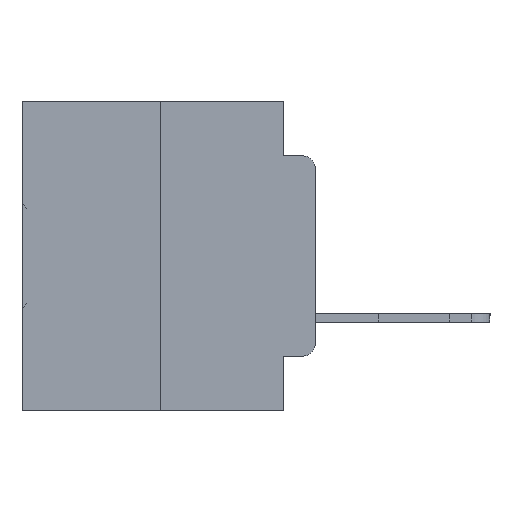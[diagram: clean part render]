
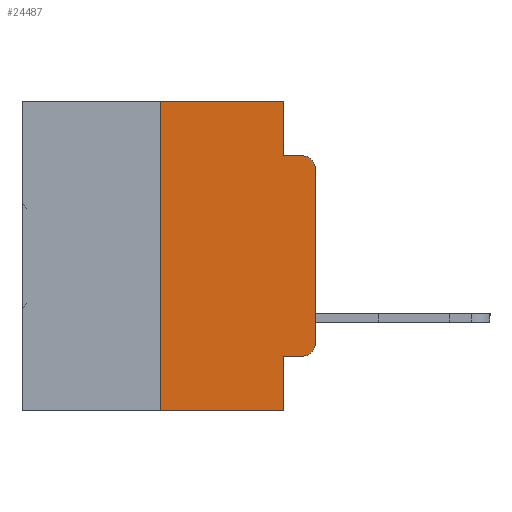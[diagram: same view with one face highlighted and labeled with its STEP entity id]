
A CAD part, left-side view. The second image highlights one B-rep face of the part: STEP entity #24487.
In plain terms, the highlighted planar face has unit normal (-1, 0, 0).
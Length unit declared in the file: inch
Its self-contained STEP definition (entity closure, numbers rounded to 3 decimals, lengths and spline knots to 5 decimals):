
#37 = VERTEX_POINT ( 'NONE', #17748 ) ;
#330 = DIRECTION ( 'NONE',  ( 0., 0., 1. ) ) ;
#816 = DIRECTION ( 'NONE',  ( 1., 0., 0. ) ) ;
#1724 = VECTOR ( 'NONE', #330, 39.37008 ) ;
#1955 = LINE ( 'NONE', #27634, #27703 ) ;
#2617 = CARTESIAN_POINT ( 'NONE',  ( 0., 0., -0.3915 ) ) ;
#2791 = LINE ( 'NONE', #24488, #22580 ) ;
#3688 = VERTEX_POINT ( 'NONE', #6544 ) ;
#3793 = FACE_OUTER_BOUND ( 'NONE', #29259, .T. ) ;
#4021 = ORIENTED_EDGE ( 'NONE', *, *, #22853, .F. ) ;
#4313 = VERTEX_POINT ( 'NONE', #27003 ) ;
#4497 = DIRECTION ( 'NONE',  ( 0., -1., 0. ) ) ;
#4817 = AXIS2_PLACEMENT_3D ( 'NONE', #11892, #29883, #14508 ) ;
#4866 = VERTEX_POINT ( 'NONE', #28330 ) ;
#6233 = CARTESIAN_POINT ( 'NONE',  ( 0., 0.473, -0.5 ) ) ;
#6544 = CARTESIAN_POINT ( 'NONE',  ( 0., 0.02, -0.4115 ) ) ;
#6559 = DIRECTION ( 'NONE',  ( 0., -1., 0. ) ) ;
#6731 = DIRECTION ( 'NONE',  ( -1., 0., 0. ) ) ;
#6744 = CARTESIAN_POINT ( 'NONE',  ( 0., 0.051, 0. ) ) ;
#7440 = LINE ( 'NONE', #6744, #33087 ) ;
#7523 = VECTOR ( 'NONE', #4497, 39.37008 ) ;
#8477 = EDGE_CURVE ( 'NONE', #4866, #23274, #1955, .T. ) ;
#9270 = DIRECTION ( 'NONE',  ( 0., 0., -1. ) ) ;
#9688 = VECTOR ( 'NONE', #19151, 39.37008 ) ;
#10139 = LINE ( 'NONE', #18176, #29871 ) ;
#10166 = EDGE_CURVE ( 'NONE', #4313, #20481, #10139, .T. ) ;
#10499 = ORIENTED_EDGE ( 'NONE', *, *, #17153, .F. ) ;
#10943 = LINE ( 'NONE', #18436, #1724 ) ;
#11037 = EDGE_CURVE ( 'NONE', #4313, #23274, #29813, .T. ) ;
#11892 = CARTESIAN_POINT ( 'NONE',  ( 0., 0.02, -0.1085 ) ) ;
#13663 = CARTESIAN_POINT ( 'NONE',  ( 0., 0.473, 0. ) ) ;
#13836 = CIRCLE ( 'NONE', #31294, 0.02 ) ;
#14319 = ORIENTED_EDGE ( 'NONE', *, *, #10166, .F. ) ;
#14508 = DIRECTION ( 'NONE',  ( 0., 0., -1. ) ) ;
#14827 = DIRECTION ( 'NONE',  ( 0., 0., -1. ) ) ;
#15124 = ORIENTED_EDGE ( 'NONE', *, *, #8477, .F. ) ;
#17153 = EDGE_CURVE ( 'NONE', #31834, #23799, #7440, .T. ) ;
#17427 = LINE ( 'NONE', #29294, #9688 ) ;
#17651 = ORIENTED_EDGE ( 'NONE', *, *, #28085, .T. ) ;
#17748 = CARTESIAN_POINT ( 'NONE',  ( 0., 0.02, -0.0885 ) ) ;
#17864 = ORIENTED_EDGE ( 'NONE', *, *, #11037, .T. ) ;
#18003 = ORIENTED_EDGE ( 'NONE', *, *, #25762, .T. ) ;
#18176 = CARTESIAN_POINT ( 'NONE',  ( 0., 0.25, 0. ) ) ;
#18436 = CARTESIAN_POINT ( 'NONE',  ( 0., 0., 0. ) ) ;
#18914 = EDGE_CURVE ( 'NONE', #23799, #37, #17427, .T. ) ;
#18917 = DIRECTION ( 'NONE',  ( 0., 0., -1. ) ) ;
#19151 = DIRECTION ( 'NONE',  ( 0., -1., 0. ) ) ;
#19980 = CARTESIAN_POINT ( 'NONE',  ( 0., 0.473, 0. ) ) ;
#20019 = ORIENTED_EDGE ( 'NONE', *, *, #29170, .T. ) ;
#20481 = VERTEX_POINT ( 'NONE', #32333 ) ;
#21280 = LINE ( 'NONE', #19980, #7523 ) ;
#21879 = AXIS2_PLACEMENT_3D ( 'NONE', #13663, #816, #18917 ) ;
#22199 = CARTESIAN_POINT ( 'NONE',  ( 0., 0.02, -0.3915 ) ) ;
#22580 = VECTOR ( 'NONE', #6559, 39.37008 ) ;
#22853 = EDGE_CURVE ( 'NONE', #20481, #31834, #21280, .T. ) ;
#23227 = DIRECTION ( 'NONE',  ( 0., 0., 1. ) ) ;
#23274 = VERTEX_POINT ( 'NONE', #29356 ) ;
#23799 = VERTEX_POINT ( 'NONE', #31423 ) ;
#23903 = VERTEX_POINT ( 'NONE', #29208 ) ;
#23922 = ORIENTED_EDGE ( 'NONE', *, *, #31494, .T. ) ;
#24487 = ADVANCED_FACE ( 'NONE', ( #3793 ), #31605, .F. ) ;
#24488 = CARTESIAN_POINT ( 'NONE',  ( 0., 0.051, -0.4115 ) ) ;
#24763 = DIRECTION ( 'NONE',  ( 0., 0., -1. ) ) ;
#25762 = EDGE_CURVE ( 'NONE', #23903, #37, #31792, .T. ) ;
#26810 = DIRECTION ( 'NONE',  ( 0., -1., 0. ) ) ;
#27003 = CARTESIAN_POINT ( 'NONE',  ( 0., 0.25, -0.5 ) ) ;
#27326 = ORIENTED_EDGE ( 'NONE', *, *, #18914, .F. ) ;
#27634 = CARTESIAN_POINT ( 'NONE',  ( 0., 0.051, 0. ) ) ;
#27703 = VECTOR ( 'NONE', #14827, 39.37008 ) ;
#28085 = EDGE_CURVE ( 'NONE', #3688, #30943, #13836, .T. ) ;
#28330 = CARTESIAN_POINT ( 'NONE',  ( 0., 0.051, -0.4115 ) ) ;
#28556 = CARTESIAN_POINT ( 'NONE',  ( 0., 0.051, 0. ) ) ;
#29013 = VECTOR ( 'NONE', #26810, 39.37008 ) ;
#29170 = EDGE_CURVE ( 'NONE', #30943, #23903, #10943, .T. ) ;
#29208 = CARTESIAN_POINT ( 'NONE',  ( 0., 0., -0.1085 ) ) ;
#29259 = EDGE_LOOP ( 'NONE', ( #20019, #18003, #27326, #10499, #4021, #14319, #17864, #15124, #23922, #17651 ) ) ;
#29294 = CARTESIAN_POINT ( 'NONE',  ( 0., 0.051, -0.0885 ) ) ;
#29356 = CARTESIAN_POINT ( 'NONE',  ( 0., 0.051, -0.5 ) ) ;
#29813 = LINE ( 'NONE', #6233, #29013 ) ;
#29871 = VECTOR ( 'NONE', #23227, 39.37008 ) ;
#29883 = DIRECTION ( 'NONE',  ( -1., 0., 0. ) ) ;
#30943 = VERTEX_POINT ( 'NONE', #2617 ) ;
#31294 = AXIS2_PLACEMENT_3D ( 'NONE', #22199, #6731, #24763 ) ;
#31423 = CARTESIAN_POINT ( 'NONE',  ( 0., 0.051, -0.0885 ) ) ;
#31494 = EDGE_CURVE ( 'NONE', #4866, #3688, #2791, .T. ) ;
#31605 = PLANE ( 'NONE',  #21879 ) ;
#31792 = CIRCLE ( 'NONE', #4817, 0.02 ) ;
#31834 = VERTEX_POINT ( 'NONE', #28556 ) ;
#32333 = CARTESIAN_POINT ( 'NONE',  ( 0., 0.25, 0. ) ) ;
#33087 = VECTOR ( 'NONE', #9270, 39.37008 ) ;
